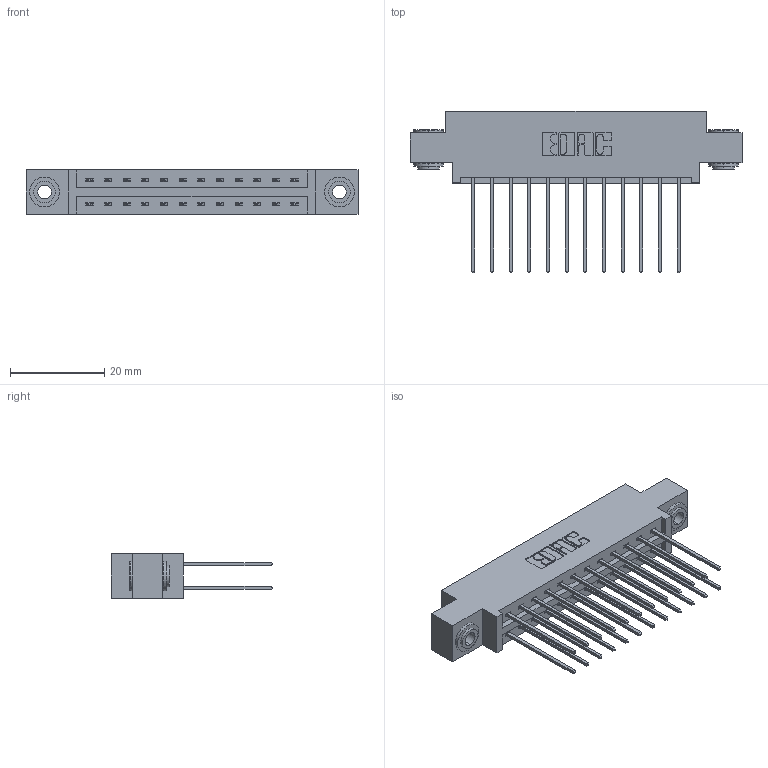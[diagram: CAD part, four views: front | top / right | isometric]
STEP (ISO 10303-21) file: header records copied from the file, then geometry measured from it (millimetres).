
FILE_DESCRIPTION (( 'STEP AP203' ), '1' );
FILE_NAME ('387-024-541-803.STEP', '2019-10-16T18:21:44', ( '' ), ( '' ), 'SwSTEP 2.0', 'SolidWorks 2016', '' );
FILE_SCHEMA (( 'CONFIG_CONTROL_DESIGN' ));
Length unit declared in the file: inch
Products named in the file (4): 345-250-002_345-250-002-102; 337 Part_0.170 Offset - 0.156 Dia-TH; 345-292-001_345-293-141; 387-024-541-803
Assembly tree (27 placements, depth 2):
  387-024-541-803
    337 Part_0.170 Offset - 0.156 Dia-TH
    345-292-001_345-293-141  x24
    345-250-002_345-250-002-102  x2
Bounding box: 70.56 x 34.3 x 9.4 mm (x, y, z)
Volume: 7076.5 mm3; surface area: 8732 mm2
Topology: 27 solids, 27 shells, 1452 faces, 4263 edges, 2806 vertices
Faces by surface type: plane 996, cylinder 448, cone 8
Entity records: 13984 total; most frequent: CARTESIAN_POINT 2357, ORIENTED_EDGE 2286, DIRECTION 2093, EDGE_CURVE 1143, VECTOR 991, LINE 991, VERTEX_POINT 758, AXIS2_PLACEMENT_3D 551
